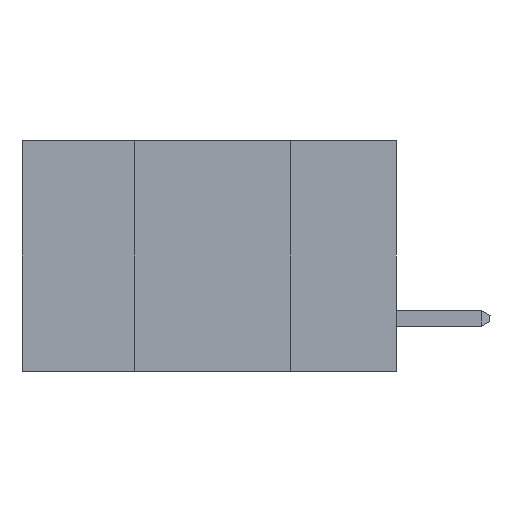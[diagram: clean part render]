
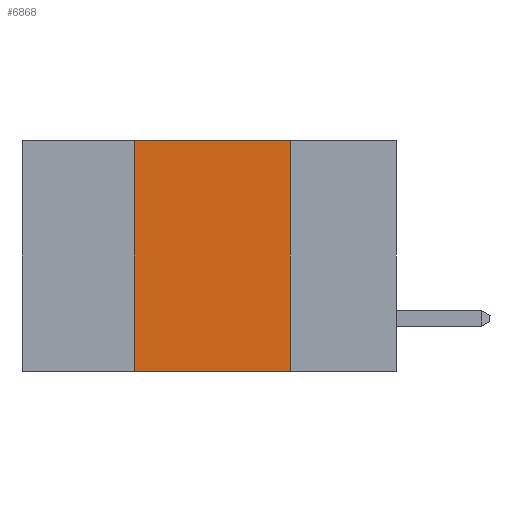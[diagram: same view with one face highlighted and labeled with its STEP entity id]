
A CAD part, left-side view. The second image highlights one B-rep face of the part: STEP entity #6868.
In plain terms, the highlighted planar face has unit normal (-1, 0, 0).
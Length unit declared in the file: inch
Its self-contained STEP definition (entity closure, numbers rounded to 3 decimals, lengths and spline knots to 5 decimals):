
#544 = CARTESIAN_POINT ( 'NONE',  ( 0., 0.6, 0. ) ) ;
#764 = EDGE_CURVE ( 'NONE', #12639, #15954, #9024, .T. ) ;
#1158 = VECTOR ( 'NONE', #6387, 39.37008 ) ;
#1183 = LINE ( 'NONE', #7836, #11837 ) ;
#1586 = VERTEX_POINT ( 'NONE', #14454 ) ;
#1906 = DIRECTION ( 'NONE',  ( 0., 0., 1. ) ) ;
#2329 = ORIENTED_EDGE ( 'NONE', *, *, #3569, .F. ) ;
#2669 = VECTOR ( 'NONE', #18696, 39.37008 ) ;
#2926 = LINE ( 'NONE', #18206, #3472 ) ;
#3472 = VECTOR ( 'NONE', #1906, 39.37008 ) ;
#3569 = EDGE_CURVE ( 'NONE', #1586, #12639, #9267, .T. ) ;
#4058 = ORIENTED_EDGE ( 'NONE', *, *, #11209, .T. ) ;
#5776 = DIRECTION ( 'NONE',  ( 0., -1., 0. ) ) ;
#6387 = DIRECTION ( 'NONE',  ( 0., -1., 0. ) ) ;
#6816 = VERTEX_POINT ( 'NONE', #19791 ) ;
#6868 = ADVANCED_FACE ( 'NONE', ( #13409 ), #14941, .F. ) ;
#6888 = DIRECTION ( 'NONE',  ( 0., 0., -1. ) ) ;
#7233 = EDGE_LOOP ( 'NONE', ( #8477, #2329, #7287, #4058 ) ) ;
#7287 = ORIENTED_EDGE ( 'NONE', *, *, #19292, .F. ) ;
#7836 = CARTESIAN_POINT ( 'NONE',  ( 0., 0.6, -0.37 ) ) ;
#8415 = AXIS2_PLACEMENT_3D ( 'NONE', #544, #15076, #6888 ) ;
#8477 = ORIENTED_EDGE ( 'NONE', *, *, #764, .F. ) ;
#8626 = CARTESIAN_POINT ( 'NONE',  ( 0., 0.17, 0. ) ) ;
#9024 = LINE ( 'NONE', #18442, #2669 ) ;
#9267 = LINE ( 'NONE', #16307, #1158 ) ;
#11209 = EDGE_CURVE ( 'NONE', #6816, #15954, #1183, .T. ) ;
#11837 = VECTOR ( 'NONE', #5776, 39.37008 ) ;
#12639 = VERTEX_POINT ( 'NONE', #8626 ) ;
#13409 = FACE_OUTER_BOUND ( 'NONE', #7233, .T. ) ;
#14454 = CARTESIAN_POINT ( 'NONE',  ( 0., 0.42, 0. ) ) ;
#14941 = PLANE ( 'NONE',  #8415 ) ;
#15076 = DIRECTION ( 'NONE',  ( 1., 0., 0. ) ) ;
#15954 = VERTEX_POINT ( 'NONE', #16817 ) ;
#16307 = CARTESIAN_POINT ( 'NONE',  ( 0., 0.6, 0. ) ) ;
#16817 = CARTESIAN_POINT ( 'NONE',  ( 0., 0.17, -0.37 ) ) ;
#18206 = CARTESIAN_POINT ( 'NONE',  ( 0., 0.42, 0. ) ) ;
#18442 = CARTESIAN_POINT ( 'NONE',  ( 0., 0.17, 0. ) ) ;
#18696 = DIRECTION ( 'NONE',  ( 0., 0., -1. ) ) ;
#19292 = EDGE_CURVE ( 'NONE', #6816, #1586, #2926, .T. ) ;
#19791 = CARTESIAN_POINT ( 'NONE',  ( 0., 0.42, -0.37 ) ) ;
